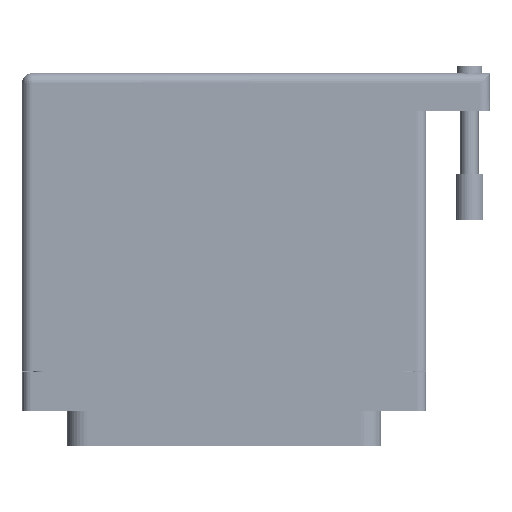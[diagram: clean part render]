
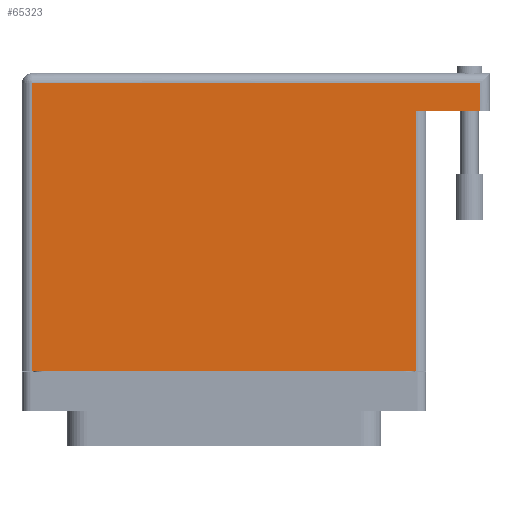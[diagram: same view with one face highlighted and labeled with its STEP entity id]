
A CAD part, front view. The second image highlights one B-rep face of the part: STEP entity #65323.
In plain terms, the highlighted face is planar.
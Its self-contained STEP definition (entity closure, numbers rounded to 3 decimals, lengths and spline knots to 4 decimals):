
#1699 = EDGE_CURVE ( 'NONE', #28326, #37587, #35659, .T. ) ;
#4476 = ORIENTED_EDGE ( 'NONE', *, *, #49451, .T. ) ;
#6440 = EDGE_CURVE ( 'NONE', #28326, #62057, #78428, .T. ) ;
#8256 = DIRECTION ( 'NONE',  ( 0., 0., -1. ) ) ;
#8561 = DIRECTION ( 'NONE',  ( -1., 0., 0. ) ) ;
#9534 = EDGE_CURVE ( 'NONE', #72808, #75317, #20198, .T. ) ;
#10518 = ORIENTED_EDGE ( 'NONE', *, *, #1699, .T. ) ;
#12478 = CARTESIAN_POINT ( 'NONE',  ( 1.3075, 1.674, 0.765 ) ) ;
#13693 = LINE ( 'NONE', #43660, #87604 ) ;
#14470 = CARTESIAN_POINT ( 'NONE',  ( 1.8125, 1.674, 0.765 ) ) ;
#20198 = LINE ( 'NONE', #21590, #62829 ) ;
#21590 = CARTESIAN_POINT ( 'NONE',  ( -1.3075, -0.1, 0.765 ) ) ;
#23806 = CARTESIAN_POINT ( 'NONE',  ( 1.3075, -0.1, 0.765 ) ) ;
#23898 = DIRECTION ( 'NONE',  ( 0., 1., 0. ) ) ;
#25598 = VECTOR ( 'NONE', #25660, 39.3701 ) ;
#25660 = DIRECTION ( 'NONE',  ( -1., 0., 0. ) ) ;
#27001 = EDGE_LOOP ( 'NONE', ( #4476, #34612, #50778, #10518, #39909, #58144 ) ) ;
#28326 = VERTEX_POINT ( 'NONE', #39010 ) ;
#34612 = ORIENTED_EDGE ( 'NONE', *, *, #35476, .T. ) ;
#35476 = EDGE_CURVE ( 'NONE', #85322, #62057, #48770, .T. ) ;
#35659 = LINE ( 'NONE', #88926, #71421 ) ;
#35697 = LINE ( 'NONE', #67308, #25598 ) ;
#35818 = DIRECTION ( 'NONE',  ( -1., 0., 0. ) ) ;
#37587 = VERTEX_POINT ( 'NONE', #70339 ) ;
#39010 = CARTESIAN_POINT ( 'NONE',  ( 1.7425, 1.674, 0.765 ) ) ;
#39163 = EDGE_CURVE ( 'NONE', #37587, #72808, #35697, .T. ) ;
#39909 = ORIENTED_EDGE ( 'NONE', *, *, #39163, .T. ) ;
#43660 = CARTESIAN_POINT ( 'NONE',  ( -1.3775, -0.1, 0.765 ) ) ;
#43980 = DIRECTION ( 'NONE',  ( 1., 0., 0. ) ) ;
#46236 = AXIS2_PLACEMENT_3D ( 'NONE', #59204, #8256, #8561 ) ;
#48770 = LINE ( 'NONE', #74020, #85678 ) ;
#49193 = DIRECTION ( 'NONE',  ( 0., -1., 0. ) ) ;
#49451 = EDGE_CURVE ( 'NONE', #75317, #85322, #13693, .T. ) ;
#50778 = ORIENTED_EDGE ( 'NONE', *, *, #6440, .F. ) ;
#56248 = CARTESIAN_POINT ( 'NONE',  ( -1.3075, 1.86, 0.765 ) ) ;
#58144 = ORIENTED_EDGE ( 'NONE', *, *, #9534, .T. ) ;
#59204 = CARTESIAN_POINT ( 'NONE',  ( -1.3775, 1.93, 0.765 ) ) ;
#62057 = VERTEX_POINT ( 'NONE', #12478 ) ;
#62829 = VECTOR ( 'NONE', #49193, 39.3701 ) ;
#65323 = ADVANCED_FACE ( 'NONE', ( #79751 ), #66411, .F. ) ;
#66411 = PLANE ( 'NONE',  #46236 ) ;
#67308 = CARTESIAN_POINT ( 'NONE',  ( -1.3775, 1.86, 0.765 ) ) ;
#70339 = CARTESIAN_POINT ( 'NONE',  ( 1.7425, 1.86, 0.765 ) ) ;
#70529 = CARTESIAN_POINT ( 'NONE',  ( -1.3075, -0.1, 0.765 ) ) ;
#71421 = VECTOR ( 'NONE', #81495, 39.3701 ) ;
#72808 = VERTEX_POINT ( 'NONE', #56248 ) ;
#74020 = CARTESIAN_POINT ( 'NONE',  ( 1.3075, 1.674, 0.765 ) ) ;
#75317 = VERTEX_POINT ( 'NONE', #70529 ) ;
#78428 = LINE ( 'NONE', #14470, #84002 ) ;
#79751 = FACE_OUTER_BOUND ( 'NONE', #27001, .T. ) ;
#81495 = DIRECTION ( 'NONE',  ( 0., 1., 0. ) ) ;
#84002 = VECTOR ( 'NONE', #35818, 39.3701 ) ;
#85322 = VERTEX_POINT ( 'NONE', #23806 ) ;
#85678 = VECTOR ( 'NONE', #23898, 39.3701 ) ;
#87604 = VECTOR ( 'NONE', #43980, 39.3701 ) ;
#88926 = CARTESIAN_POINT ( 'NONE',  ( 1.7425, 1.93, 0.765 ) ) ;
